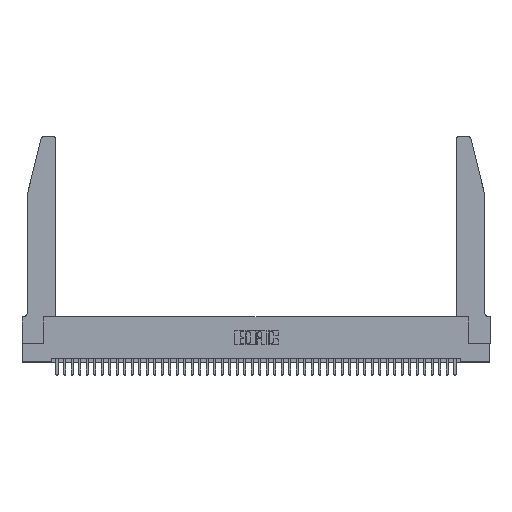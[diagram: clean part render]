
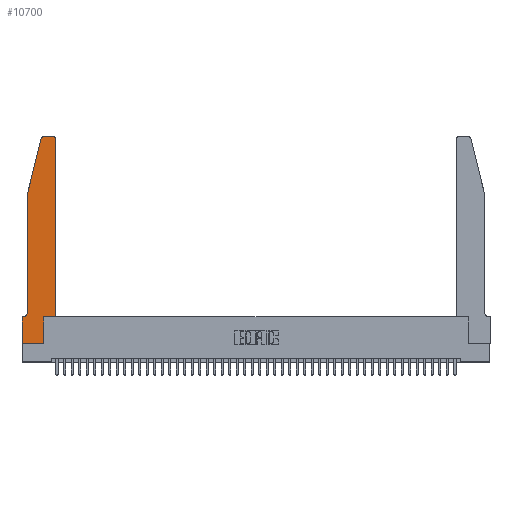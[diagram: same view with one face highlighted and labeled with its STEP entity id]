
A CAD part, top view. The second image highlights one B-rep face of the part: STEP entity #10700.
In plain terms, the highlighted planar face has unit normal (0, 0, 1).
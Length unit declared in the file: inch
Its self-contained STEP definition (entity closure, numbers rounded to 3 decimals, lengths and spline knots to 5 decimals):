
#48 = CARTESIAN_POINT ( 'NONE',  ( 0.0755, 2., 0.37 ) ) ;
#841 = AXIS2_PLACEMENT_3D ( 'NONE', #2280, #9369, #16461 ) ;
#899 = DIRECTION ( 'NONE',  ( -1., 0., 0. ) ) ;
#1005 = ORIENTED_EDGE ( 'NONE', *, *, #44719, .T. ) ;
#1101 = ORIENTED_EDGE ( 'NONE', *, *, #18094, .T. ) ;
#2280 = CARTESIAN_POINT ( 'NONE',  ( 0.0055, 0.42, 0.37 ) ) ;
#3257 = EDGE_CURVE ( 'NONE', #16084, #5077, #15582, .T. ) ;
#3607 = VECTOR ( 'NONE', #39891, 39.37008 ) ;
#3788 = VERTEX_POINT ( 'NONE', #13233 ) ;
#3863 = ORIENTED_EDGE ( 'NONE', *, *, #3257, .T. ) ;
#5077 = VERTEX_POINT ( 'NONE', #21686 ) ;
#5252 = CARTESIAN_POINT ( 'NONE',  ( 0., 0.35, 0.37 ) ) ;
#5276 = CARTESIAN_POINT ( 'NONE',  ( 0.0055, 0.35, 0.37 ) ) ;
#5394 = EDGE_CURVE ( 'NONE', #14585, #9361, #24743, .T. ) ;
#5694 = EDGE_LOOP ( 'NONE', ( #15857, #1005, #40666, #22647, #15965, #33880, #37553, #7391, #1101, #39333, #3863, #28944 ) ) ;
#5799 = CARTESIAN_POINT ( 'NONE',  ( 0.284, 2.75, 0.37 ) ) ;
#7304 = VECTOR ( 'NONE', #37703, 39.37008 ) ;
#7391 = ORIENTED_EDGE ( 'NONE', *, *, #32175, .T. ) ;
#7575 = VECTOR ( 'NONE', #24675, 39.37008 ) ;
#8718 = LINE ( 'NONE', #48, #7575 ) ;
#9361 = VERTEX_POINT ( 'NONE', #9863 ) ;
#9369 = DIRECTION ( 'NONE',  ( 0., 0., -1. ) ) ;
#9842 = CARTESIAN_POINT ( 'NONE',  ( 0.0755, 0.35, 0.37 ) ) ;
#9863 = CARTESIAN_POINT ( 'NONE',  ( 0., 0., 0.37 ) ) ;
#10097 = LINE ( 'NONE', #23145, #37107 ) ;
#10301 = DIRECTION ( 'NONE',  ( -0.239, -0.971, 0. ) ) ;
#10559 = VERTEX_POINT ( 'NONE', #5276 ) ;
#10700 = ADVANCED_FACE ( 'NONE', ( #34855 ), #26357, .T. ) ;
#10975 = VERTEX_POINT ( 'NONE', #24175 ) ;
#12591 = LINE ( 'NONE', #35987, #42335 ) ;
#12972 = CIRCLE ( 'NONE', #14457, 0.03 ) ;
#13223 = CIRCLE ( 'NONE', #32001, 0.03 ) ;
#13233 = CARTESIAN_POINT ( 'NONE',  ( 0.2865, 0.35, 0.37 ) ) ;
#13672 = CARTESIAN_POINT ( 'NONE',  ( 0.25487, 2.72718, 0.37 ) ) ;
#14283 = VECTOR ( 'NONE', #30636, 39.37008 ) ;
#14457 = AXIS2_PLACEMENT_3D ( 'NONE', #16019, #29865, #37104 ) ;
#14585 = VERTEX_POINT ( 'NONE', #30723 ) ;
#15582 = LINE ( 'NONE', #33991, #7304 ) ;
#15739 = CARTESIAN_POINT ( 'NONE',  ( 0.4205, 2.72, 0.37 ) ) ;
#15857 = ORIENTED_EDGE ( 'NONE', *, *, #22314, .T. ) ;
#15965 = ORIENTED_EDGE ( 'NONE', *, *, #21523, .T. ) ;
#16019 = CARTESIAN_POINT ( 'NONE',  ( 0.284, 2.72, 0.37 ) ) ;
#16084 = VERTEX_POINT ( 'NONE', #41867 ) ;
#16461 = DIRECTION ( 'NONE',  ( -1., 0., 0. ) ) ;
#17253 = EDGE_CURVE ( 'NONE', #10559, #14585, #23206, .T. ) ;
#18094 = EDGE_CURVE ( 'NONE', #10975, #3788, #26448, .T. ) ;
#18210 = VERTEX_POINT ( 'NONE', #13672 ) ;
#18775 = CARTESIAN_POINT ( 'NONE',  ( 0., 0., 0.37 ) ) ;
#18790 = DIRECTION ( 'NONE',  ( 1., 0., 0. ) ) ;
#18880 = EDGE_CURVE ( 'NONE', #24179, #34581, #8718, .T. ) ;
#19618 = EDGE_CURVE ( 'NONE', #3788, #16084, #12591, .T. ) ;
#20107 = CIRCLE ( 'NONE', #841, 0.07 ) ;
#21046 = AXIS2_PLACEMENT_3D ( 'NONE', #5252, #39903, #18790 ) ;
#21523 = EDGE_CURVE ( 'NONE', #34581, #10559, #20107, .T. ) ;
#21686 = CARTESIAN_POINT ( 'NONE',  ( 0.4505, 2.72, 0.37 ) ) ;
#22314 = EDGE_CURVE ( 'NONE', #22590, #43735, #26669, .T. ) ;
#22325 = EDGE_CURVE ( 'NONE', #18210, #24179, #10097, .T. ) ;
#22590 = VERTEX_POINT ( 'NONE', #36831 ) ;
#22647 = ORIENTED_EDGE ( 'NONE', *, *, #18880, .T. ) ;
#22754 = VECTOR ( 'NONE', #899, 39.37008 ) ;
#23145 = CARTESIAN_POINT ( 'NONE',  ( 0.0755, 2., 0.37 ) ) ;
#23206 = LINE ( 'NONE', #9842, #24327 ) ;
#24175 = CARTESIAN_POINT ( 'NONE',  ( 0.2865, 0., 0.37 ) ) ;
#24179 = VERTEX_POINT ( 'NONE', #42336 ) ;
#24327 = VECTOR ( 'NONE', #27809, 39.37008 ) ;
#24675 = DIRECTION ( 'NONE',  ( 0., -1., 0. ) ) ;
#24743 = LINE ( 'NONE', #26951, #14283 ) ;
#25639 = DIRECTION ( 'NONE',  ( 1., 0., 0. ) ) ;
#26173 = DIRECTION ( 'NONE',  ( 0., 0., 1. ) ) ;
#26357 = PLANE ( 'NONE',  #21046 ) ;
#26448 = LINE ( 'NONE', #39578, #28092 ) ;
#26669 = LINE ( 'NONE', #41106, #22754 ) ;
#26951 = CARTESIAN_POINT ( 'NONE',  ( 0., 0., 0.37 ) ) ;
#27809 = DIRECTION ( 'NONE',  ( -1., 0., 0. ) ) ;
#28092 = VECTOR ( 'NONE', #42993, 39.37008 ) ;
#28944 = ORIENTED_EDGE ( 'NONE', *, *, #36241, .T. ) ;
#29865 = DIRECTION ( 'NONE',  ( 0., 0., 1. ) ) ;
#30636 = DIRECTION ( 'NONE',  ( 0., -1., 0. ) ) ;
#30723 = CARTESIAN_POINT ( 'NONE',  ( 0., 0.35, 0.37 ) ) ;
#31346 = CARTESIAN_POINT ( 'NONE',  ( 0.0755, 0.42, 0.37 ) ) ;
#32001 = AXIS2_PLACEMENT_3D ( 'NONE', #15739, #26173, #44106 ) ;
#32175 = EDGE_CURVE ( 'NONE', #9361, #10975, #44485, .T. ) ;
#33880 = ORIENTED_EDGE ( 'NONE', *, *, #17253, .T. ) ;
#33991 = CARTESIAN_POINT ( 'NONE',  ( 0.4505, 0.35, 0.37 ) ) ;
#34581 = VERTEX_POINT ( 'NONE', #31346 ) ;
#34855 = FACE_OUTER_BOUND ( 'NONE', #5694, .T. ) ;
#35987 = CARTESIAN_POINT ( 'NONE',  ( 0.4505, 0.35, 0.37 ) ) ;
#36241 = EDGE_CURVE ( 'NONE', #5077, #22590, #13223, .T. ) ;
#36831 = CARTESIAN_POINT ( 'NONE',  ( 0.4205, 2.75, 0.37 ) ) ;
#37104 = DIRECTION ( 'NONE',  ( 1., 0., 0. ) ) ;
#37107 = VECTOR ( 'NONE', #10301, 39.37008 ) ;
#37553 = ORIENTED_EDGE ( 'NONE', *, *, #5394, .T. ) ;
#37703 = DIRECTION ( 'NONE',  ( 0., 1., 0. ) ) ;
#39333 = ORIENTED_EDGE ( 'NONE', *, *, #19618, .T. ) ;
#39578 = CARTESIAN_POINT ( 'NONE',  ( 0.2865, 0.35, 0.37 ) ) ;
#39891 = DIRECTION ( 'NONE',  ( 1., 0., 0. ) ) ;
#39903 = DIRECTION ( 'NONE',  ( 0., 0., 1. ) ) ;
#40666 = ORIENTED_EDGE ( 'NONE', *, *, #22325, .T. ) ;
#41106 = CARTESIAN_POINT ( 'NONE',  ( 0.2605, 2.75, 0.37 ) ) ;
#41867 = CARTESIAN_POINT ( 'NONE',  ( 0.4505, 0.35, 0.37 ) ) ;
#42335 = VECTOR ( 'NONE', #25639, 39.37008 ) ;
#42336 = CARTESIAN_POINT ( 'NONE',  ( 0.0755, 2., 0.37 ) ) ;
#42993 = DIRECTION ( 'NONE',  ( 0., 1., 0. ) ) ;
#43735 = VERTEX_POINT ( 'NONE', #5799 ) ;
#44106 = DIRECTION ( 'NONE',  ( 1., 0., 0. ) ) ;
#44485 = LINE ( 'NONE', #18775, #3607 ) ;
#44719 = EDGE_CURVE ( 'NONE', #43735, #18210, #12972, .T. ) ;
